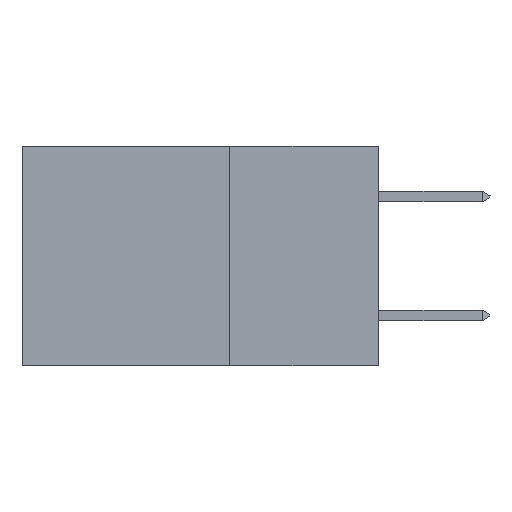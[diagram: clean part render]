
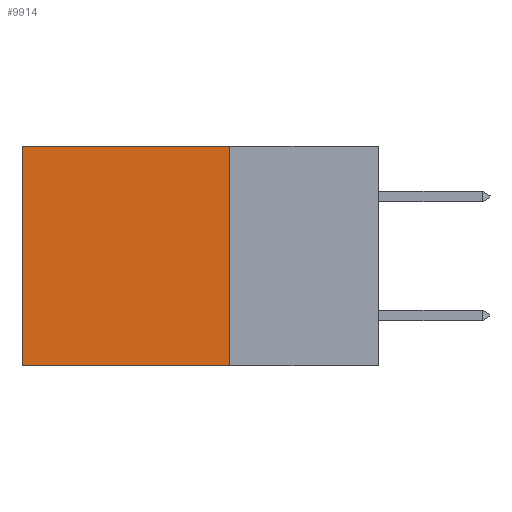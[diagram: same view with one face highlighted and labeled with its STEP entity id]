
A CAD part, left-side view. The second image highlights one B-rep face of the part: STEP entity #9914.
In plain terms, the highlighted planar face has unit normal (-1, 0, 0).
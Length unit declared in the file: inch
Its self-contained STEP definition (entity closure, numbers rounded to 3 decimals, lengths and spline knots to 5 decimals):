
#606 = CARTESIAN_POINT ( 'NONE',  ( 0.2615, 0.25, -0.37 ) ) ;
#1922 = EDGE_LOOP ( 'NONE', ( #3240, #3470, #1934, #9212 ) ) ;
#1934 = ORIENTED_EDGE ( 'NONE', *, *, #6157, .F. ) ;
#2027 = VERTEX_POINT ( 'NONE', #3362 ) ;
#2039 = VECTOR ( 'NONE', #8440, 39.37008 ) ;
#2107 = CARTESIAN_POINT ( 'NONE',  ( 0.2615, 0.25, -0.37 ) ) ;
#2214 = VERTEX_POINT ( 'NONE', #9338 ) ;
#2351 = DIRECTION ( 'NONE',  ( 0., 0., -1. ) ) ;
#2432 = VECTOR ( 'NONE', #4120, 39.37008 ) ;
#3240 = ORIENTED_EDGE ( 'NONE', *, *, #6408, .T. ) ;
#3243 = VERTEX_POINT ( 'NONE', #7615 ) ;
#3362 = CARTESIAN_POINT ( 'NONE',  ( 0.2615, 0.25, 0. ) ) ;
#3470 = ORIENTED_EDGE ( 'NONE', *, *, #9585, .F. ) ;
#3976 = VECTOR ( 'NONE', #9538, 39.37008 ) ;
#4120 = DIRECTION ( 'NONE',  ( 0., 1., 0. ) ) ;
#4341 = CARTESIAN_POINT ( 'NONE',  ( 0.2615, 0.6, -0.37 ) ) ;
#4712 = CARTESIAN_POINT ( 'NONE',  ( 0.2615, 0.25, -0.37 ) ) ;
#4807 = LINE ( 'NONE', #4912, #2432 ) ;
#4912 = CARTESIAN_POINT ( 'NONE',  ( 0.2615, 0.25, 0. ) ) ;
#5277 = LINE ( 'NONE', #4341, #2039 ) ;
#6157 = EDGE_CURVE ( 'NONE', #2027, #2214, #6354, .T. ) ;
#6319 = VECTOR ( 'NONE', #8006, 39.37008 ) ;
#6354 = LINE ( 'NONE', #4712, #3976 ) ;
#6360 = PLANE ( 'NONE',  #9317 ) ;
#6408 = EDGE_CURVE ( 'NONE', #10034, #3243, #5277, .T. ) ;
#7615 = CARTESIAN_POINT ( 'NONE',  ( 0.2615, 0.6, -0.37 ) ) ;
#7797 = LINE ( 'NONE', #606, #6319 ) ;
#7933 = DIRECTION ( 'NONE',  ( 1., 0., 0. ) ) ;
#8006 = DIRECTION ( 'NONE',  ( 0., 1., 0. ) ) ;
#8440 = DIRECTION ( 'NONE',  ( 0., 0., -1. ) ) ;
#9149 = EDGE_CURVE ( 'NONE', #2027, #10034, #4807, .T. ) ;
#9197 = FACE_OUTER_BOUND ( 'NONE', #1922, .T. ) ;
#9212 = ORIENTED_EDGE ( 'NONE', *, *, #9149, .T. ) ;
#9317 = AXIS2_PLACEMENT_3D ( 'NONE', #2107, #7933, #2351 ) ;
#9338 = CARTESIAN_POINT ( 'NONE',  ( 0.2615, 0.25, -0.37 ) ) ;
#9538 = DIRECTION ( 'NONE',  ( 0., 0., -1. ) ) ;
#9585 = EDGE_CURVE ( 'NONE', #2214, #3243, #7797, .T. ) ;
#9914 = ADVANCED_FACE ( 'NONE', ( #9197 ), #6360, .F. ) ;
#10034 = VERTEX_POINT ( 'NONE', #10078 ) ;
#10078 = CARTESIAN_POINT ( 'NONE',  ( 0.2615, 0.6, 0. ) ) ;
